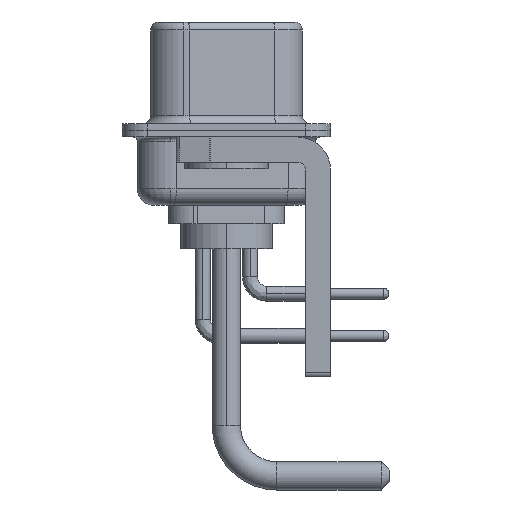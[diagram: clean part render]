
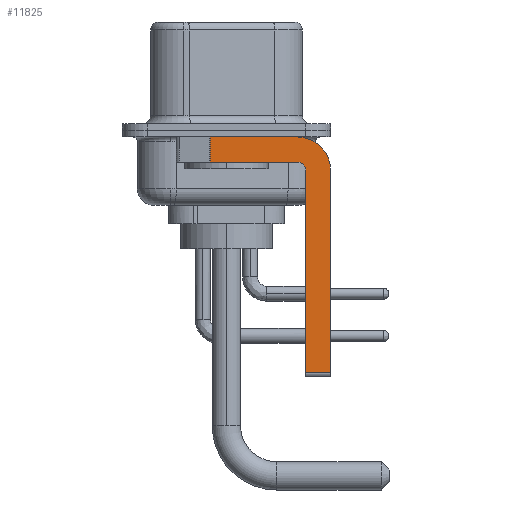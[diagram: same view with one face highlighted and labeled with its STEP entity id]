
A CAD part, left-side view. The second image highlights one B-rep face of the part: STEP entity #11825.
In plain terms, the highlighted planar face has unit normal (-1, 0, 0).
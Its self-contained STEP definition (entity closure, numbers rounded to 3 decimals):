
#735 = CARTESIAN_POINT ( 'NONE',  ( -2.9, -4.25, -14.55 ) ) ;
#1127 = VECTOR ( 'NONE', #26183, 1000. ) ;
#1738 = AXIS2_PLACEMENT_3D ( 'NONE', #16728, #8214, #10738 ) ;
#1751 = CIRCLE ( 'NONE', #23060, 2. ) ;
#1972 = DIRECTION ( 'NONE',  ( 1., 0., 0. ) ) ;
#1993 = CARTESIAN_POINT ( 'NONE',  ( -2.9, 0.978, -0.4 ) ) ;
#2517 = EDGE_CURVE ( 'NONE', #13396, #22061, #17907, .T. ) ;
#2590 = VECTOR ( 'NONE', #11386, 1000. ) ;
#2886 = CARTESIAN_POINT ( 'NONE',  ( -2.9, -4.25, -1.9 ) ) ;
#3175 = DIRECTION ( 'NONE',  ( 0., 0., -1. ) ) ;
#4270 = CIRCLE ( 'NONE', #17472, 0.5 ) ;
#4502 = VERTEX_POINT ( 'NONE', #14222 ) ;
#5003 = LINE ( 'NONE', #2886, #17892 ) ;
#5755 = CARTESIAN_POINT ( 'NONE',  ( -2.9, -6.25, -2.4 ) ) ;
#7925 = EDGE_CURVE ( 'NONE', #19331, #20244, #24040, .T. ) ;
#7984 = CARTESIAN_POINT ( 'NONE',  ( -2.9, -4.25, -2.4 ) ) ;
#8208 = VERTEX_POINT ( 'NONE', #10946 ) ;
#8214 = DIRECTION ( 'NONE',  ( 1., 0., 0. ) ) ;
#8339 = PLANE ( 'NONE',  #1738 ) ;
#8876 = DIRECTION ( 'NONE',  ( 0., -1., 0. ) ) ;
#10316 = ORIENTED_EDGE ( 'NONE', *, *, #2517, .F. ) ;
#10336 = FACE_OUTER_BOUND ( 'NONE', #14305, .T. ) ;
#10542 = ORIENTED_EDGE ( 'NONE', *, *, #21231, .F. ) ;
#10738 = DIRECTION ( 'NONE',  ( 0., 0., -1. ) ) ;
#10946 = CARTESIAN_POINT ( 'NONE',  ( -2.9, -4.75, -14.55 ) ) ;
#11386 = DIRECTION ( 'NONE',  ( 0., -1., 0. ) ) ;
#11486 = EDGE_CURVE ( 'NONE', #14643, #4502, #5003, .T. ) ;
#11545 = EDGE_CURVE ( 'NONE', #12405, #14643, #4270, .T. ) ;
#11546 = DIRECTION ( 'NONE',  ( -1., 0., 0. ) ) ;
#11609 = VECTOR ( 'NONE', #3175, 1000. ) ;
#11825 = ADVANCED_FACE ( 'NONE', ( #10336 ), #8339, .F. ) ;
#11832 = LINE ( 'NONE', #17297, #11609 ) ;
#12405 = VERTEX_POINT ( 'NONE', #16485 ) ;
#12565 = CARTESIAN_POINT ( 'NONE',  ( -2.9, -4.75, -14.8 ) ) ;
#12631 = EDGE_CURVE ( 'NONE', #8208, #20244, #15013, .T. ) ;
#12632 = ORIENTED_EDGE ( 'NONE', *, *, #11545, .F. ) ;
#13396 = VERTEX_POINT ( 'NONE', #1993 ) ;
#14222 = CARTESIAN_POINT ( 'NONE',  ( -2.9, 0.978, -1.9 ) ) ;
#14305 = EDGE_LOOP ( 'NONE', ( #10316, #19202, #23765, #12632, #22687, #22018, #19526, #10542 ) ) ;
#14643 = VERTEX_POINT ( 'NONE', #20430 ) ;
#14700 = LINE ( 'NONE', #12565, #21148 ) ;
#15013 = LINE ( 'NONE', #735, #23903 ) ;
#15248 = EDGE_CURVE ( 'NONE', #8208, #12405, #14700, .T. ) ;
#15261 = CARTESIAN_POINT ( 'NONE',  ( -2.9, -4.25, -0.4 ) ) ;
#15418 = DIRECTION ( 'NONE',  ( 0., 1., 0. ) ) ;
#15549 = CARTESIAN_POINT ( 'NONE',  ( -2.9, -4.25, -2.4 ) ) ;
#16485 = CARTESIAN_POINT ( 'NONE',  ( -2.9, -4.75, -2.4 ) ) ;
#16728 = CARTESIAN_POINT ( 'NONE',  ( -2.9, -4.25, -2.4 ) ) ;
#17297 = CARTESIAN_POINT ( 'NONE',  ( -2.9, 0.978, -1.9 ) ) ;
#17472 = AXIS2_PLACEMENT_3D ( 'NONE', #15549, #11546, #19685 ) ;
#17892 = VECTOR ( 'NONE', #15418, 1000. ) ;
#17907 = LINE ( 'NONE', #19659, #2590 ) ;
#18376 = DIRECTION ( 'NONE',  ( 0., 0., -1. ) ) ;
#19202 = ORIENTED_EDGE ( 'NONE', *, *, #23961, .T. ) ;
#19331 = VERTEX_POINT ( 'NONE', #19539 ) ;
#19526 = ORIENTED_EDGE ( 'NONE', *, *, #7925, .F. ) ;
#19539 = CARTESIAN_POINT ( 'NONE',  ( -2.9, -6.25, -2.4 ) ) ;
#19659 = CARTESIAN_POINT ( 'NONE',  ( -2.9, 3., -0.4 ) ) ;
#19685 = DIRECTION ( 'NONE',  ( 0., 0., 1. ) ) ;
#20244 = VERTEX_POINT ( 'NONE', #21279 ) ;
#20430 = CARTESIAN_POINT ( 'NONE',  ( -2.9, -4.25, -1.9 ) ) ;
#21148 = VECTOR ( 'NONE', #25110, 1000. ) ;
#21231 = EDGE_CURVE ( 'NONE', #22061, #19331, #1751, .T. ) ;
#21279 = CARTESIAN_POINT ( 'NONE',  ( -2.9, -6.25, -14.55 ) ) ;
#22018 = ORIENTED_EDGE ( 'NONE', *, *, #12631, .T. ) ;
#22061 = VERTEX_POINT ( 'NONE', #15261 ) ;
#22687 = ORIENTED_EDGE ( 'NONE', *, *, #15248, .F. ) ;
#23060 = AXIS2_PLACEMENT_3D ( 'NONE', #7984, #1972, #18376 ) ;
#23765 = ORIENTED_EDGE ( 'NONE', *, *, #11486, .F. ) ;
#23903 = VECTOR ( 'NONE', #8876, 1000. ) ;
#23961 = EDGE_CURVE ( 'NONE', #13396, #4502, #11832, .T. ) ;
#24040 = LINE ( 'NONE', #5755, #1127 ) ;
#25110 = DIRECTION ( 'NONE',  ( 0., 0., 1. ) ) ;
#26183 = DIRECTION ( 'NONE',  ( 0., 0., -1. ) ) ;
